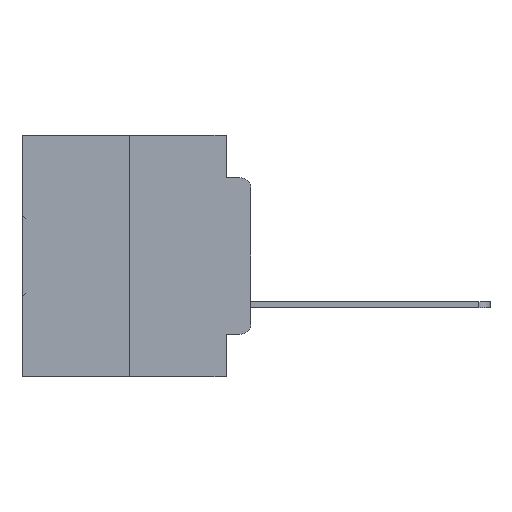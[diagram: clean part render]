
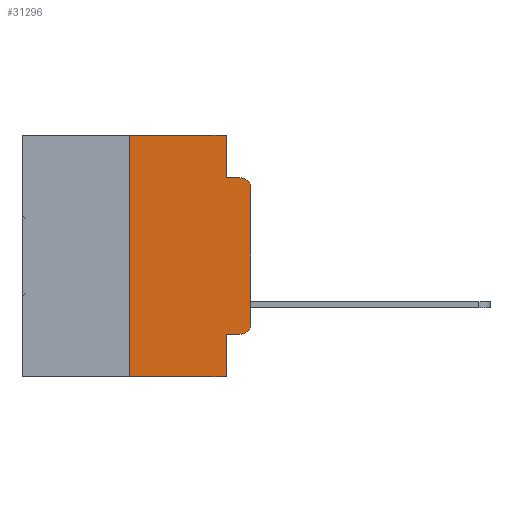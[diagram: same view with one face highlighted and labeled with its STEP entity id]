
A CAD part, left-side view. The second image highlights one B-rep face of the part: STEP entity #31296.
In plain terms, the highlighted planar face has unit normal (-1, 0, 0).
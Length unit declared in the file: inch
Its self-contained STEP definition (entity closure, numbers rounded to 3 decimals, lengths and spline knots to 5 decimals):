
#430 = CARTESIAN_POINT ( 'NONE',  ( 0., 0., 0. ) ) ;
#495 = ORIENTED_EDGE ( 'NONE', *, *, #10803, .T. ) ;
#623 = FACE_OUTER_BOUND ( 'NONE', #22062, .T. ) ;
#844 = LINE ( 'NONE', #3012, #7588 ) ;
#1786 = DIRECTION ( 'NONE',  ( 0., 0., -1. ) ) ;
#1930 = VECTOR ( 'NONE', #9142, 39.37008 ) ;
#1971 = VECTOR ( 'NONE', #1786, 39.37008 ) ;
#2419 = LINE ( 'NONE', #18772, #16208 ) ;
#3012 = CARTESIAN_POINT ( 'NONE',  ( 0., 0.473, 0. ) ) ;
#3097 = VECTOR ( 'NONE', #3765, 39.37008 ) ;
#3765 = DIRECTION ( 'NONE',  ( 0., -1., 0. ) ) ;
#4714 = CARTESIAN_POINT ( 'NONE',  ( 0., 0.051, -0.4115 ) ) ;
#6053 = EDGE_CURVE ( 'NONE', #13272, #10906, #844, .T. ) ;
#6654 = VERTEX_POINT ( 'NONE', #12418 ) ;
#7241 = DIRECTION ( 'NONE',  ( 1., 0., 0. ) ) ;
#7507 = CARTESIAN_POINT ( 'NONE',  ( 0., 0.02, -0.3915 ) ) ;
#7588 = VECTOR ( 'NONE', #21505, 39.37008 ) ;
#8232 = VERTEX_POINT ( 'NONE', #25099 ) ;
#8357 = CARTESIAN_POINT ( 'NONE',  ( 0., 0., -0.1085 ) ) ;
#9142 = DIRECTION ( 'NONE',  ( 0., -1., 0. ) ) ;
#9550 = LINE ( 'NONE', #28939, #1930 ) ;
#9654 = EDGE_CURVE ( 'NONE', #18265, #16196, #10738, .T. ) ;
#9671 = CARTESIAN_POINT ( 'NONE',  ( 0., 0.02, -0.1085 ) ) ;
#9746 = CARTESIAN_POINT ( 'NONE',  ( 0., 0.02, -0.0885 ) ) ;
#9813 = CARTESIAN_POINT ( 'NONE',  ( 0., 0.051, -0.0885 ) ) ;
#10395 = DIRECTION ( 'NONE',  ( 0., 0., -1. ) ) ;
#10512 = LINE ( 'NONE', #27618, #1971 ) ;
#10738 = LINE ( 'NONE', #19812, #3097 ) ;
#10803 = EDGE_CURVE ( 'NONE', #20940, #13286, #20107, .T. ) ;
#10902 = EDGE_CURVE ( 'NONE', #13286, #20445, #15472, .T. ) ;
#10906 = VERTEX_POINT ( 'NONE', #19948 ) ;
#10956 = EDGE_CURVE ( 'NONE', #6654, #20445, #21229, .T. ) ;
#11067 = EDGE_CURVE ( 'NONE', #10906, #6654, #10512, .T. ) ;
#11165 = EDGE_CURVE ( 'NONE', #18265, #13272, #31152, .T. ) ;
#11206 = EDGE_CURVE ( 'NONE', #17052, #16196, #2419, .T. ) ;
#11350 = EDGE_CURVE ( 'NONE', #17052, #8232, #9550, .T. ) ;
#11572 = EDGE_CURVE ( 'NONE', #8232, #20940, #21170, .T. ) ;
#11723 = CARTESIAN_POINT ( 'NONE',  ( 0., 0.051, -0.5 ) ) ;
#12418 = CARTESIAN_POINT ( 'NONE',  ( 0., 0.051, -0.0885 ) ) ;
#12492 = DIRECTION ( 'NONE',  ( 0., 0., -1. ) ) ;
#12950 = ORIENTED_EDGE ( 'NONE', *, *, #11572, .T. ) ;
#13272 = VERTEX_POINT ( 'NONE', #23533 ) ;
#13286 = VERTEX_POINT ( 'NONE', #8357 ) ;
#15472 = CIRCLE ( 'NONE', #28318, 0.02 ) ;
#16196 = VERTEX_POINT ( 'NONE', #11723 ) ;
#16208 = VECTOR ( 'NONE', #32929, 39.37008 ) ;
#17052 = VERTEX_POINT ( 'NONE', #4714 ) ;
#17687 = DIRECTION ( 'NONE',  ( 0., -1., 0. ) ) ;
#17857 = PLANE ( 'NONE',  #26102 ) ;
#17908 = CARTESIAN_POINT ( 'NONE',  ( 0., 0., -0.3915 ) ) ;
#18265 = VERTEX_POINT ( 'NONE', #23047 ) ;
#18460 = ORIENTED_EDGE ( 'NONE', *, *, #11067, .F. ) ;
#18555 = CARTESIAN_POINT ( 'NONE',  ( 0., 0.25, 0. ) ) ;
#18772 = CARTESIAN_POINT ( 'NONE',  ( 0., 0.051, 0. ) ) ;
#19812 = CARTESIAN_POINT ( 'NONE',  ( 0., 0.473, -0.5 ) ) ;
#19948 = CARTESIAN_POINT ( 'NONE',  ( 0., 0.051, 0. ) ) ;
#20107 = LINE ( 'NONE', #430, #31878 ) ;
#20445 = VERTEX_POINT ( 'NONE', #9746 ) ;
#20940 = VERTEX_POINT ( 'NONE', #17908 ) ;
#20995 = DIRECTION ( 'NONE',  ( 0., 0., 1. ) ) ;
#21170 = CIRCLE ( 'NONE', #22368, 0.02 ) ;
#21229 = LINE ( 'NONE', #9813, #26778 ) ;
#21505 = DIRECTION ( 'NONE',  ( 0., -1., 0. ) ) ;
#21852 = DIRECTION ( 'NONE',  ( 0., 0., 1. ) ) ;
#22062 = EDGE_LOOP ( 'NONE', ( #495, #28885, #22586, #18460, #25599, #31768, #32466, #29259, #30005, #12950 ) ) ;
#22368 = AXIS2_PLACEMENT_3D ( 'NONE', #7507, #25328, #10395 ) ;
#22586 = ORIENTED_EDGE ( 'NONE', *, *, #10956, .F. ) ;
#22701 = CARTESIAN_POINT ( 'NONE',  ( 0., 0.473, 0. ) ) ;
#23047 = CARTESIAN_POINT ( 'NONE',  ( 0., 0.25, -0.5 ) ) ;
#23533 = CARTESIAN_POINT ( 'NONE',  ( 0., 0.25, 0. ) ) ;
#25099 = CARTESIAN_POINT ( 'NONE',  ( 0., 0.02, -0.4115 ) ) ;
#25120 = DIRECTION ( 'NONE',  ( 0., 0., -1. ) ) ;
#25328 = DIRECTION ( 'NONE',  ( -1., 0., 0. ) ) ;
#25599 = ORIENTED_EDGE ( 'NONE', *, *, #6053, .F. ) ;
#25685 = VECTOR ( 'NONE', #20995, 39.37008 ) ;
#26102 = AXIS2_PLACEMENT_3D ( 'NONE', #22701, #7241, #25120 ) ;
#26778 = VECTOR ( 'NONE', #17687, 39.37008 ) ;
#27105 = DIRECTION ( 'NONE',  ( -1., 0., 0. ) ) ;
#27618 = CARTESIAN_POINT ( 'NONE',  ( 0., 0.051, 0. ) ) ;
#28318 = AXIS2_PLACEMENT_3D ( 'NONE', #9671, #27105, #12492 ) ;
#28885 = ORIENTED_EDGE ( 'NONE', *, *, #10902, .T. ) ;
#28939 = CARTESIAN_POINT ( 'NONE',  ( 0., 0.051, -0.4115 ) ) ;
#29259 = ORIENTED_EDGE ( 'NONE', *, *, #11206, .F. ) ;
#30005 = ORIENTED_EDGE ( 'NONE', *, *, #11350, .T. ) ;
#31152 = LINE ( 'NONE', #18555, #25685 ) ;
#31296 = ADVANCED_FACE ( 'NONE', ( #623 ), #17857, .F. ) ;
#31768 = ORIENTED_EDGE ( 'NONE', *, *, #11165, .F. ) ;
#31878 = VECTOR ( 'NONE', #21852, 39.37008 ) ;
#32466 = ORIENTED_EDGE ( 'NONE', *, *, #9654, .T. ) ;
#32929 = DIRECTION ( 'NONE',  ( 0., 0., -1. ) ) ;
